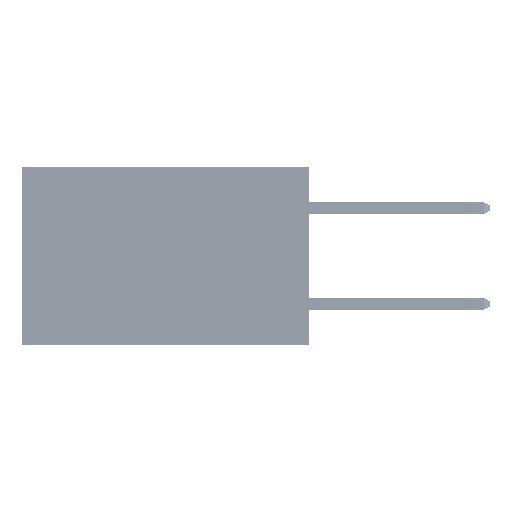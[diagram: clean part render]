
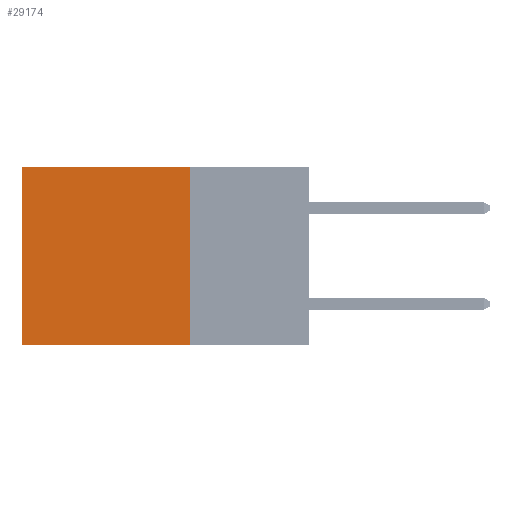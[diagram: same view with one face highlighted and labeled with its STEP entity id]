
A CAD part, left-side view. The second image highlights one B-rep face of the part: STEP entity #29174.
In plain terms, the highlighted planar face has unit normal (-1, 0, 0).
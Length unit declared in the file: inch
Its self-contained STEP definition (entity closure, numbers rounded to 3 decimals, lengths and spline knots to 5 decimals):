
#270 = AXIS2_PLACEMENT_3D ( 'NONE', #20892, #46141, #29093 ) ;
#1302 = LINE ( 'NONE', #17159, #22709 ) ;
#1500 = LINE ( 'NONE', #2579, #23527 ) ;
#2042 = VERTEX_POINT ( 'NONE', #13247 ) ;
#2065 = CARTESIAN_POINT ( 'NONE',  ( 0.2875, 0.25, -0.37 ) ) ;
#2579 = CARTESIAN_POINT ( 'NONE',  ( 0.2875, 0.25, 0. ) ) ;
#4672 = EDGE_CURVE ( 'NONE', #2042, #25382, #46266, .T. ) ;
#5684 = ORIENTED_EDGE ( 'NONE', *, *, #14285, .F. ) ;
#5846 = EDGE_CURVE ( 'NONE', #21174, #2042, #1302, .T. ) ;
#9590 = VERTEX_POINT ( 'NONE', #33762 ) ;
#13182 = DIRECTION ( 'NONE',  ( 0., 1., 0. ) ) ;
#13247 = CARTESIAN_POINT ( 'NONE',  ( 0.2875, 0.6, 0. ) ) ;
#14285 = EDGE_CURVE ( 'NONE', #21174, #9590, #1500, .T. ) ;
#15390 = FACE_OUTER_BOUND ( 'NONE', #53049, .T. ) ;
#16668 = VECTOR ( 'NONE', #51575, 39.37008 ) ;
#17159 = CARTESIAN_POINT ( 'NONE',  ( 0.2875, 0.25, 0. ) ) ;
#19913 = CARTESIAN_POINT ( 'NONE',  ( 0.2875, 0.6, -0.37 ) ) ;
#20892 = CARTESIAN_POINT ( 'NONE',  ( 0.2875, 0.25, 0. ) ) ;
#21174 = VERTEX_POINT ( 'NONE', #47493 ) ;
#21705 = ORIENTED_EDGE ( 'NONE', *, *, #4672, .T. ) ;
#22537 = CARTESIAN_POINT ( 'NONE',  ( 0.2875, 0.6, 0. ) ) ;
#22709 = VECTOR ( 'NONE', #13182, 39.37008 ) ;
#23527 = VECTOR ( 'NONE', #27402, 39.37008 ) ;
#24277 = ORIENTED_EDGE ( 'NONE', *, *, #5846, .T. ) ;
#25382 = VERTEX_POINT ( 'NONE', #19913 ) ;
#27402 = DIRECTION ( 'NONE',  ( 0., 0., -1. ) ) ;
#27728 = LINE ( 'NONE', #2065, #16668 ) ;
#29093 = DIRECTION ( 'NONE',  ( 0., 0., -1. ) ) ;
#29174 = ADVANCED_FACE ( 'NONE', ( #15390 ), #37968, .F. ) ;
#33762 = CARTESIAN_POINT ( 'NONE',  ( 0.2875, 0.25, -0.37 ) ) ;
#34535 = ORIENTED_EDGE ( 'NONE', *, *, #43941, .F. ) ;
#37823 = VECTOR ( 'NONE', #43392, 39.37008 ) ;
#37968 = PLANE ( 'NONE',  #270 ) ;
#43392 = DIRECTION ( 'NONE',  ( 0., 0., -1. ) ) ;
#43941 = EDGE_CURVE ( 'NONE', #9590, #25382, #27728, .T. ) ;
#46141 = DIRECTION ( 'NONE',  ( 1., 0., 0. ) ) ;
#46266 = LINE ( 'NONE', #22537, #37823 ) ;
#47493 = CARTESIAN_POINT ( 'NONE',  ( 0.2875, 0.25, 0. ) ) ;
#51575 = DIRECTION ( 'NONE',  ( 0., 1., 0. ) ) ;
#53049 = EDGE_LOOP ( 'NONE', ( #21705, #34535, #5684, #24277 ) ) ;
